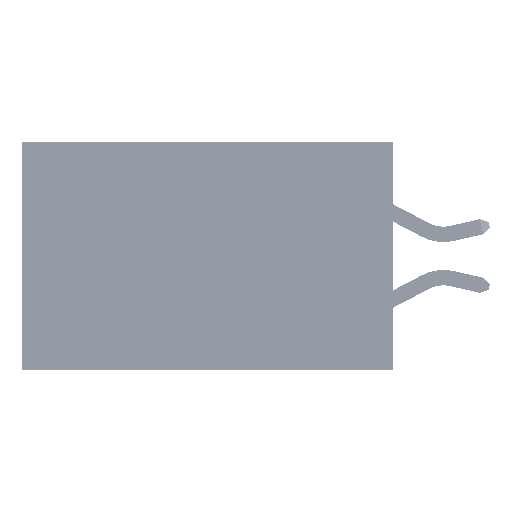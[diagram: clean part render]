
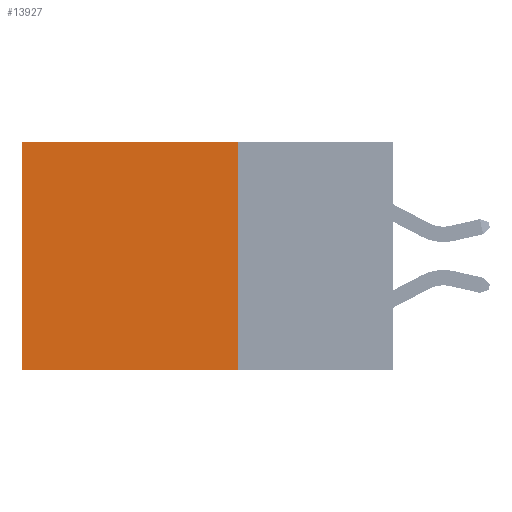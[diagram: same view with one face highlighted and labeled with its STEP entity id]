
A CAD part, left-side view. The second image highlights one B-rep face of the part: STEP entity #13927.
In plain terms, the highlighted planar face has unit normal (-1, 0, 0).
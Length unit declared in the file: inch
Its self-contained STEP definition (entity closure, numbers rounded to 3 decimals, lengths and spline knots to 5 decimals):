
#3075 = DIRECTION ( 'NONE',  ( 0., 1., 0. ) ) ;
#5429 = CARTESIAN_POINT ( 'NONE',  ( 0.2875, 0.25, -0.37 ) ) ;
#6386 = LINE ( 'NONE', #5429, #10783 ) ;
#6512 = EDGE_CURVE ( 'NONE', #10002, #15866, #6386, .T. ) ;
#9512 = DIRECTION ( 'NONE',  ( 0., 0., -1. ) ) ;
#10002 = VERTEX_POINT ( 'NONE', #50964 ) ;
#10783 = VECTOR ( 'NONE', #17058, 39.37008 ) ;
#13756 = VERTEX_POINT ( 'NONE', #17150 ) ;
#13927 = ADVANCED_FACE ( 'NONE', ( #26126 ), #34126, .F. ) ;
#15866 = VERTEX_POINT ( 'NONE', #31079 ) ;
#17058 = DIRECTION ( 'NONE',  ( 0., 1., 0. ) ) ;
#17150 = CARTESIAN_POINT ( 'NONE',  ( 0.2875, 0.25, 0. ) ) ;
#17329 = ORIENTED_EDGE ( 'NONE', *, *, #20803, .T. ) ;
#20803 = EDGE_CURVE ( 'NONE', #13756, #30151, #44776, .T. ) ;
#23297 = EDGE_CURVE ( 'NONE', #13756, #10002, #26480, .T. ) ;
#24303 = DIRECTION ( 'NONE',  ( 0., 0., -1. ) ) ;
#26126 = FACE_OUTER_BOUND ( 'NONE', #42297, .T. ) ;
#26480 = LINE ( 'NONE', #48551, #28363 ) ;
#28363 = VECTOR ( 'NONE', #24303, 39.37008 ) ;
#29036 = EDGE_CURVE ( 'NONE', #30151, #15866, #30861, .T. ) ;
#30151 = VERTEX_POINT ( 'NONE', #47941 ) ;
#30270 = DIRECTION ( 'NONE',  ( 1., 0., 0. ) ) ;
#30838 = CARTESIAN_POINT ( 'NONE',  ( 0.2875, 0.25, 0. ) ) ;
#30861 = LINE ( 'NONE', #33737, #38415 ) ;
#31079 = CARTESIAN_POINT ( 'NONE',  ( 0.2875, 0.6, -0.37 ) ) ;
#33737 = CARTESIAN_POINT ( 'NONE',  ( 0.2875, 0.6, 0. ) ) ;
#33781 = DIRECTION ( 'NONE',  ( 0., 0., -1. ) ) ;
#34061 = VECTOR ( 'NONE', #3075, 39.37008 ) ;
#34126 = PLANE ( 'NONE',  #45949 ) ;
#34304 = CARTESIAN_POINT ( 'NONE',  ( 0.2875, 0.25, 0. ) ) ;
#38415 = VECTOR ( 'NONE', #9512, 39.37008 ) ;
#41423 = ORIENTED_EDGE ( 'NONE', *, *, #29036, .T. ) ;
#42297 = EDGE_LOOP ( 'NONE', ( #41423, #46364, #44289, #17329 ) ) ;
#44289 = ORIENTED_EDGE ( 'NONE', *, *, #23297, .F. ) ;
#44776 = LINE ( 'NONE', #30838, #34061 ) ;
#45949 = AXIS2_PLACEMENT_3D ( 'NONE', #34304, #30270, #33781 ) ;
#46364 = ORIENTED_EDGE ( 'NONE', *, *, #6512, .F. ) ;
#47941 = CARTESIAN_POINT ( 'NONE',  ( 0.2875, 0.6, 0. ) ) ;
#48551 = CARTESIAN_POINT ( 'NONE',  ( 0.2875, 0.25, 0. ) ) ;
#50964 = CARTESIAN_POINT ( 'NONE',  ( 0.2875, 0.25, -0.37 ) ) ;
